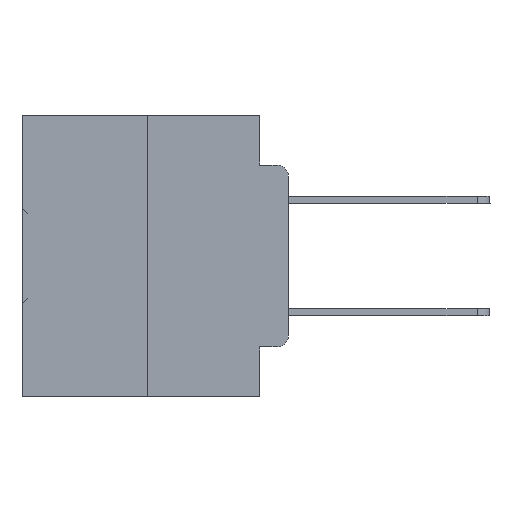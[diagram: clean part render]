
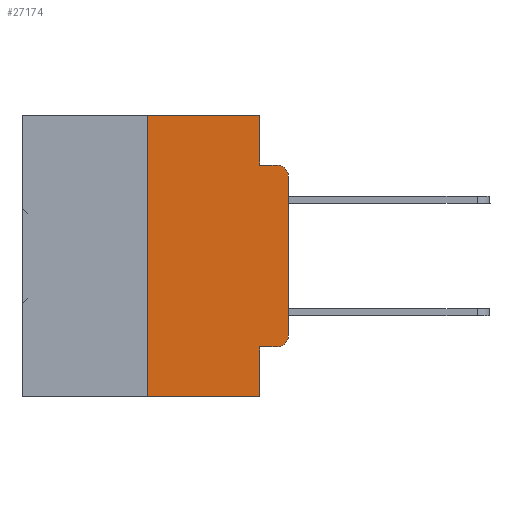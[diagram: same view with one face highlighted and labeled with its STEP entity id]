
A CAD part, left-side view. The second image highlights one B-rep face of the part: STEP entity #27174.
In plain terms, the highlighted planar face has unit normal (-1, 0, 0).
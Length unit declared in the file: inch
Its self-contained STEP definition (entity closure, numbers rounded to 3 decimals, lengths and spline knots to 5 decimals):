
#963 = EDGE_CURVE ( 'NONE', #38838, #31933, #31047, .T. ) ;
#1750 = DIRECTION ( 'NONE',  ( 1., 0., 0. ) ) ;
#1862 = CARTESIAN_POINT ( 'NONE',  ( 0., 0.051, -0.4115 ) ) ;
#3365 = VERTEX_POINT ( 'NONE', #22131 ) ;
#3636 = LINE ( 'NONE', #24696, #7540 ) ;
#4581 = LINE ( 'NONE', #7775, #14700 ) ;
#5362 = EDGE_CURVE ( 'NONE', #31178, #37039, #3636, .T. ) ;
#6465 = LINE ( 'NONE', #9260, #13859 ) ;
#7119 = DIRECTION ( 'NONE',  ( 0., 0., -1. ) ) ;
#7374 = AXIS2_PLACEMENT_3D ( 'NONE', #17033, #1750, #7119 ) ;
#7540 = VECTOR ( 'NONE', #15540, 39.37008 ) ;
#7775 = CARTESIAN_POINT ( 'NONE',  ( 0., 0.051, 0. ) ) ;
#7906 = FACE_OUTER_BOUND ( 'NONE', #37808, .T. ) ;
#8023 = LINE ( 'NONE', #1862, #30124 ) ;
#8414 = EDGE_CURVE ( 'NONE', #35392, #37039, #21503, .T. ) ;
#9260 = CARTESIAN_POINT ( 'NONE',  ( 0., 0.473, 0. ) ) ;
#9364 = CARTESIAN_POINT ( 'NONE',  ( 0., 0.051, 0. ) ) ;
#9719 = CARTESIAN_POINT ( 'NONE',  ( 0., 0., 0. ) ) ;
#9965 = CARTESIAN_POINT ( 'NONE',  ( 0., 0.02, -0.3915 ) ) ;
#10510 = VECTOR ( 'NONE', #35016, 39.37008 ) ;
#11254 = ORIENTED_EDGE ( 'NONE', *, *, #31208, .F. ) ;
#11269 = CARTESIAN_POINT ( 'NONE',  ( 0., 0.25, -0.5 ) ) ;
#11388 = DIRECTION ( 'NONE',  ( 0., -1., 0. ) ) ;
#11995 = ORIENTED_EDGE ( 'NONE', *, *, #22844, .T. ) ;
#13133 = DIRECTION ( 'NONE',  ( 0., 0., -1. ) ) ;
#13576 = CARTESIAN_POINT ( 'NONE',  ( 0., 0.051, -0.5 ) ) ;
#13859 = VECTOR ( 'NONE', #21399, 39.37008 ) ;
#13910 = AXIS2_PLACEMENT_3D ( 'NONE', #9965, #37615, #13133 ) ;
#14700 = VECTOR ( 'NONE', #19714, 39.37008 ) ;
#15372 = CARTESIAN_POINT ( 'NONE',  ( 0., 0.051, -0.0885 ) ) ;
#15540 = DIRECTION ( 'NONE',  ( 0., -1., 0. ) ) ;
#15595 = AXIS2_PLACEMENT_3D ( 'NONE', #19525, #30838, #21904 ) ;
#15665 = LINE ( 'NONE', #9719, #17510 ) ;
#16152 = ORIENTED_EDGE ( 'NONE', *, *, #38806, .T. ) ;
#16534 = VERTEX_POINT ( 'NONE', #20581 ) ;
#17033 = CARTESIAN_POINT ( 'NONE',  ( 0., 0.473, 0. ) ) ;
#17305 = ORIENTED_EDGE ( 'NONE', *, *, #5362, .T. ) ;
#17310 = EDGE_CURVE ( 'NONE', #25753, #35566, #4581, .T. ) ;
#17510 = VECTOR ( 'NONE', #27794, 39.37008 ) ;
#18746 = VECTOR ( 'NONE', #36812, 39.37008 ) ;
#18973 = ORIENTED_EDGE ( 'NONE', *, *, #38593, .F. ) ;
#18996 = ORIENTED_EDGE ( 'NONE', *, *, #35778, .T. ) ;
#19438 = CIRCLE ( 'NONE', #15595, 0.02 ) ;
#19525 = CARTESIAN_POINT ( 'NONE',  ( 0., 0.02, -0.1085 ) ) ;
#19714 = DIRECTION ( 'NONE',  ( 0., 0., -1. ) ) ;
#19923 = CARTESIAN_POINT ( 'NONE',  ( 0., 0.051, 0. ) ) ;
#20156 = EDGE_CURVE ( 'NONE', #35566, #16534, #36141, .T. ) ;
#20581 = CARTESIAN_POINT ( 'NONE',  ( 0., 0.02, -0.0885 ) ) ;
#21207 = CARTESIAN_POINT ( 'NONE',  ( 0., 0.02, -0.4115 ) ) ;
#21399 = DIRECTION ( 'NONE',  ( 0., -1., 0. ) ) ;
#21503 = LINE ( 'NONE', #9364, #18746 ) ;
#21904 = DIRECTION ( 'NONE',  ( 0., 0., -1. ) ) ;
#22131 = CARTESIAN_POINT ( 'NONE',  ( 0., 0., -0.1085 ) ) ;
#22370 = ORIENTED_EDGE ( 'NONE', *, *, #20156, .F. ) ;
#22429 = ORIENTED_EDGE ( 'NONE', *, *, #963, .T. ) ;
#22844 = EDGE_CURVE ( 'NONE', #3365, #16534, #19438, .T. ) ;
#23646 = CARTESIAN_POINT ( 'NONE',  ( 0., 0., -0.3915 ) ) ;
#24696 = CARTESIAN_POINT ( 'NONE',  ( 0., 0.473, -0.5 ) ) ;
#25753 = VERTEX_POINT ( 'NONE', #19923 ) ;
#27174 = ADVANCED_FACE ( 'NONE', ( #7906 ), #37738, .F. ) ;
#27188 = ORIENTED_EDGE ( 'NONE', *, *, #8414, .F. ) ;
#27694 = CARTESIAN_POINT ( 'NONE',  ( 0., 0.25, 0. ) ) ;
#27794 = DIRECTION ( 'NONE',  ( 0., 0., 1. ) ) ;
#29241 = ORIENTED_EDGE ( 'NONE', *, *, #17310, .F. ) ;
#29489 = VECTOR ( 'NONE', #30535, 39.37008 ) ;
#30124 = VECTOR ( 'NONE', #11388, 39.37008 ) ;
#30535 = DIRECTION ( 'NONE',  ( 0., -1., 0. ) ) ;
#30838 = DIRECTION ( 'NONE',  ( -1., 0., 0. ) ) ;
#31047 = CIRCLE ( 'NONE', #13910, 0.02 ) ;
#31178 = VERTEX_POINT ( 'NONE', #11269 ) ;
#31208 = EDGE_CURVE ( 'NONE', #34396, #25753, #6465, .T. ) ;
#31933 = VERTEX_POINT ( 'NONE', #23646 ) ;
#33721 = CARTESIAN_POINT ( 'NONE',  ( 0., 0.051, -0.0885 ) ) ;
#34396 = VERTEX_POINT ( 'NONE', #27694 ) ;
#34812 = LINE ( 'NONE', #37431, #10510 ) ;
#35016 = DIRECTION ( 'NONE',  ( 0., 0., 1. ) ) ;
#35392 = VERTEX_POINT ( 'NONE', #38883 ) ;
#35566 = VERTEX_POINT ( 'NONE', #15372 ) ;
#35778 = EDGE_CURVE ( 'NONE', #35392, #38838, #8023, .T. ) ;
#36141 = LINE ( 'NONE', #33721, #29489 ) ;
#36812 = DIRECTION ( 'NONE',  ( 0., 0., -1. ) ) ;
#37039 = VERTEX_POINT ( 'NONE', #13576 ) ;
#37431 = CARTESIAN_POINT ( 'NONE',  ( 0., 0.25, 0. ) ) ;
#37615 = DIRECTION ( 'NONE',  ( -1., 0., 0. ) ) ;
#37738 = PLANE ( 'NONE',  #7374 ) ;
#37808 = EDGE_LOOP ( 'NONE', ( #16152, #11995, #22370, #29241, #11254, #18973, #17305, #27188, #18996, #22429 ) ) ;
#38593 = EDGE_CURVE ( 'NONE', #31178, #34396, #34812, .T. ) ;
#38806 = EDGE_CURVE ( 'NONE', #31933, #3365, #15665, .T. ) ;
#38838 = VERTEX_POINT ( 'NONE', #21207 ) ;
#38883 = CARTESIAN_POINT ( 'NONE',  ( 0., 0.051, -0.4115 ) ) ;
